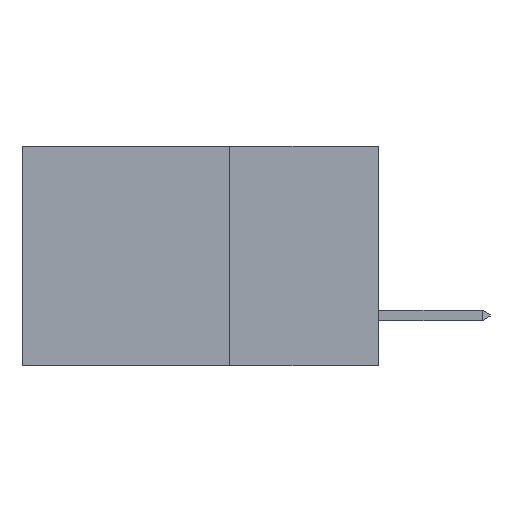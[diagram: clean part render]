
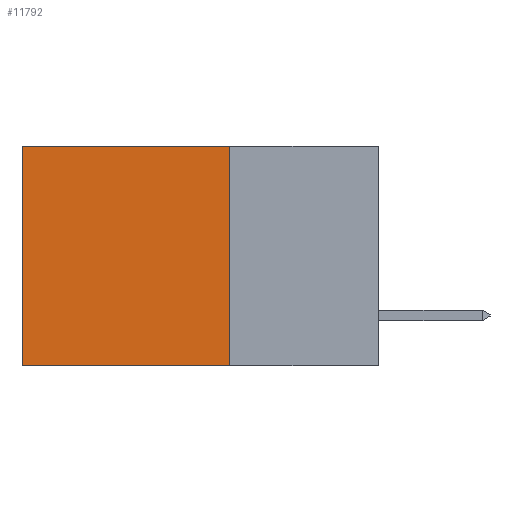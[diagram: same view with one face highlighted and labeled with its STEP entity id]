
A CAD part, left-side view. The second image highlights one B-rep face of the part: STEP entity #11792.
In plain terms, the highlighted planar face has unit normal (-1, 0, 0).
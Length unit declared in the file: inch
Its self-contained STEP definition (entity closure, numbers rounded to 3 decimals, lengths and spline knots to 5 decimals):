
#95 = CARTESIAN_POINT ( 'NONE',  ( 0.2615, 0.25, -0.37 ) ) ;
#163 = FACE_OUTER_BOUND ( 'NONE', #888, .T. ) ;
#229 = LINE ( 'NONE', #8109, #5601 ) ;
#279 = VERTEX_POINT ( 'NONE', #1861 ) ;
#433 = VERTEX_POINT ( 'NONE', #5952 ) ;
#604 = DIRECTION ( 'NONE',  ( 0., 0., -1. ) ) ;
#656 = CARTESIAN_POINT ( 'NONE',  ( 0.2615, 0.6, -0.37 ) ) ;
#888 = EDGE_LOOP ( 'NONE', ( #9428, #10761, #10624, #9445 ) ) ;
#900 = EDGE_CURVE ( 'NONE', #2188, #433, #5785, .T. ) ;
#1043 = EDGE_CURVE ( 'NONE', #2188, #279, #229, .T. ) ;
#1455 = AXIS2_PLACEMENT_3D ( 'NONE', #9164, #11956, #6196 ) ;
#1588 = CARTESIAN_POINT ( 'NONE',  ( 0.2615, 0.25, -0.37 ) ) ;
#1861 = CARTESIAN_POINT ( 'NONE',  ( 0.2615, 0.6, 0. ) ) ;
#1885 = DIRECTION ( 'NONE',  ( 0., 0., -1. ) ) ;
#2151 = EDGE_CURVE ( 'NONE', #433, #10143, #9196, .T. ) ;
#2188 = VERTEX_POINT ( 'NONE', #12579 ) ;
#3273 = EDGE_CURVE ( 'NONE', #279, #10143, #9896, .T. ) ;
#5131 = PLANE ( 'NONE',  #1455 ) ;
#5601 = VECTOR ( 'NONE', #7511, 39.37008 ) ;
#5785 = LINE ( 'NONE', #1588, #10661 ) ;
#5952 = CARTESIAN_POINT ( 'NONE',  ( 0.2615, 0.25, -0.37 ) ) ;
#6196 = DIRECTION ( 'NONE',  ( 0., 0., -1. ) ) ;
#6565 = VECTOR ( 'NONE', #12977, 39.37008 ) ;
#7311 = VECTOR ( 'NONE', #604, 39.37008 ) ;
#7511 = DIRECTION ( 'NONE',  ( 0., 1., 0. ) ) ;
#8109 = CARTESIAN_POINT ( 'NONE',  ( 0.2615, 0.25, 0. ) ) ;
#9164 = CARTESIAN_POINT ( 'NONE',  ( 0.2615, 0.25, -0.37 ) ) ;
#9196 = LINE ( 'NONE', #95, #6565 ) ;
#9428 = ORIENTED_EDGE ( 'NONE', *, *, #3273, .T. ) ;
#9445 = ORIENTED_EDGE ( 'NONE', *, *, #1043, .T. ) ;
#9896 = LINE ( 'NONE', #656, #7311 ) ;
#10143 = VERTEX_POINT ( 'NONE', #12507 ) ;
#10624 = ORIENTED_EDGE ( 'NONE', *, *, #900, .F. ) ;
#10661 = VECTOR ( 'NONE', #1885, 39.37008 ) ;
#10761 = ORIENTED_EDGE ( 'NONE', *, *, #2151, .F. ) ;
#11792 = ADVANCED_FACE ( 'NONE', ( #163 ), #5131, .F. ) ;
#11956 = DIRECTION ( 'NONE',  ( 1., 0., 0. ) ) ;
#12507 = CARTESIAN_POINT ( 'NONE',  ( 0.2615, 0.6, -0.37 ) ) ;
#12579 = CARTESIAN_POINT ( 'NONE',  ( 0.2615, 0.25, 0. ) ) ;
#12977 = DIRECTION ( 'NONE',  ( 0., 1., 0. ) ) ;
